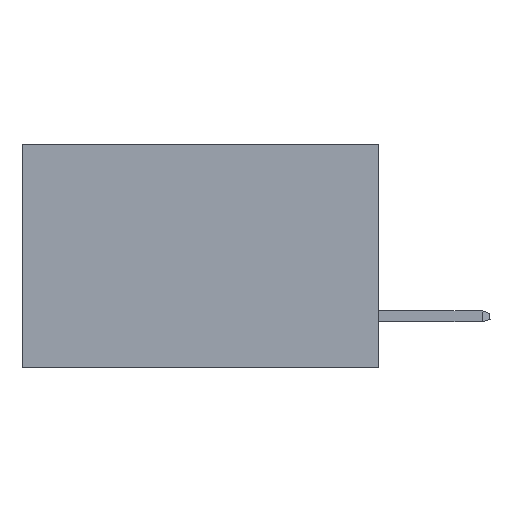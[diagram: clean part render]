
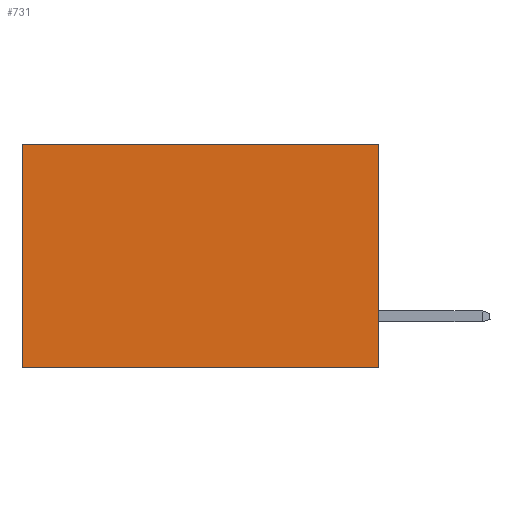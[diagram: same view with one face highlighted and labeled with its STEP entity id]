
A CAD part, left-side view. The second image highlights one B-rep face of the part: STEP entity #731.
In plain terms, the highlighted planar face has unit normal (-1, 0, 0).
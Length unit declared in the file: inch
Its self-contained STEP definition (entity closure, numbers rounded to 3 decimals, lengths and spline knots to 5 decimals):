
#255 = LINE ( 'NONE', #13018, #6135 ) ;
#617 = VERTEX_POINT ( 'NONE', #7497 ) ;
#620 = DIRECTION ( 'NONE',  ( 0., 0., -1. ) ) ;
#689 = CARTESIAN_POINT ( 'NONE',  ( 0.277, 0.59, -0.37 ) ) ;
#731 = ADVANCED_FACE ( 'NONE', ( #4722 ), #1371, .F. ) ;
#1371 = PLANE ( 'NONE',  #6052 ) ;
#1395 = CARTESIAN_POINT ( 'NONE',  ( 0.277, 0., -0.37 ) ) ;
#1701 = DIRECTION ( 'NONE',  ( 0., 1., 0. ) ) ;
#1926 = DIRECTION ( 'NONE',  ( 1., 0., 0. ) ) ;
#1939 = DIRECTION ( 'NONE',  ( 0., 0., -1. ) ) ;
#2474 = VECTOR ( 'NONE', #1701, 39.37008 ) ;
#2979 = EDGE_LOOP ( 'NONE', ( #7068, #11830, #4305, #12680 ) ) ;
#3054 = VERTEX_POINT ( 'NONE', #10918 ) ;
#3095 = EDGE_CURVE ( 'NONE', #617, #3054, #255, .T. ) ;
#3265 = VECTOR ( 'NONE', #620, 39.37008 ) ;
#3600 = CARTESIAN_POINT ( 'NONE',  ( 0.277, 0.59, -0.37 ) ) ;
#4305 = ORIENTED_EDGE ( 'NONE', *, *, #14425, .F. ) ;
#4464 = VERTEX_POINT ( 'NONE', #3600 ) ;
#4722 = FACE_OUTER_BOUND ( 'NONE', #2979, .T. ) ;
#5101 = EDGE_CURVE ( 'NONE', #3054, #4464, #8540, .T. ) ;
#5542 = LINE ( 'NONE', #9711, #2474 ) ;
#6052 = AXIS2_PLACEMENT_3D ( 'NONE', #1395, #1926, #1939 ) ;
#6135 = VECTOR ( 'NONE', #9182, 39.37008 ) ;
#6544 = VERTEX_POINT ( 'NONE', #11199 ) ;
#7068 = ORIENTED_EDGE ( 'NONE', *, *, #5101, .T. ) ;
#7308 = DIRECTION ( 'NONE',  ( 0., 0., -1. ) ) ;
#7497 = CARTESIAN_POINT ( 'NONE',  ( 0.277, 0., 0. ) ) ;
#8540 = LINE ( 'NONE', #689, #3265 ) ;
#9182 = DIRECTION ( 'NONE',  ( 0., 1., 0. ) ) ;
#9235 = LINE ( 'NONE', #12956, #12271 ) ;
#9711 = CARTESIAN_POINT ( 'NONE',  ( 0.277, 0., -0.37 ) ) ;
#10272 = EDGE_CURVE ( 'NONE', #6544, #4464, #5542, .T. ) ;
#10918 = CARTESIAN_POINT ( 'NONE',  ( 0.277, 0.59, 0. ) ) ;
#11199 = CARTESIAN_POINT ( 'NONE',  ( 0.277, 0., -0.37 ) ) ;
#11830 = ORIENTED_EDGE ( 'NONE', *, *, #10272, .F. ) ;
#12271 = VECTOR ( 'NONE', #7308, 39.37008 ) ;
#12680 = ORIENTED_EDGE ( 'NONE', *, *, #3095, .T. ) ;
#12956 = CARTESIAN_POINT ( 'NONE',  ( 0.277, 0., -0.37 ) ) ;
#13018 = CARTESIAN_POINT ( 'NONE',  ( 0.277, 0., 0. ) ) ;
#14425 = EDGE_CURVE ( 'NONE', #617, #6544, #9235, .T. ) ;
